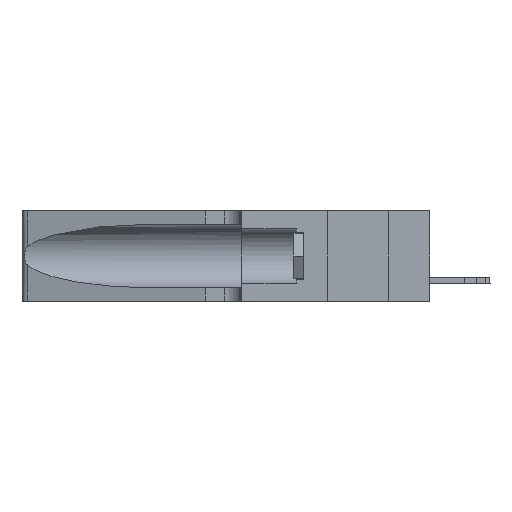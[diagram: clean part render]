
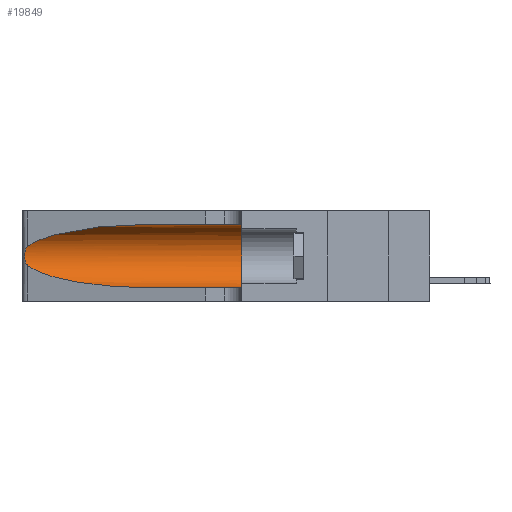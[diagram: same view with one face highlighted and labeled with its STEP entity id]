
A CAD part, left-side view. The second image highlights one B-rep face of the part: STEP entity #19849.
In plain terms, the highlighted cylindrical face has radius 3.308 mm (diameter 6.617 mm), a partial arc.
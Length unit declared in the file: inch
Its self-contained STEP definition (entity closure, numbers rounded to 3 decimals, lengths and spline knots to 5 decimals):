
#324 = CARTESIAN_POINT ( 'NONE',  ( 0.1305, 0.35, 0.31525 ) ) ;
#595 = CARTESIAN_POINT ( 'NONE',  ( 0.25856, 1.23593, 0.16098 ) ) ;
#1309 = CYLINDRICAL_SURFACE ( 'NONE', #14048, 0.13025 ) ;
#1411 = AXIS2_PLACEMENT_3D ( 'NONE', #2124, #25890, #4333 ) ;
#1624 = EDGE_CURVE ( 'NONE', #9108, #6388, #1844, .T. ) ;
#1844 = CIRCLE ( 'NONE', #1411, 0.13025 ) ;
#2124 = CARTESIAN_POINT ( 'NONE',  ( 0.1305, 0.35, 0.185 ) ) ;
#2140 = EDGE_CURVE ( 'NONE', #6096, #9663, #15116, .T. ) ;
#2176 = EDGE_CURVE ( 'NONE', #9663, #3178, #10924, .T. ) ;
#2189 = CARTESIAN_POINT ( 'NONE',  ( 0.1305, 0.72297, 0.05475 ) ) ;
#2686 = CARTESIAN_POINT ( 'NONE',  ( 0.25555, 1.22994, 0.2215 ) ) ;
#3178 = VERTEX_POINT ( 'NONE', #6890 ) ;
#3411 = CARTESIAN_POINT ( 'NONE',  ( 0.1305, 0.72297, 0.31525 ) ) ;
#4243 = EDGE_LOOP ( 'NONE', ( #12942, #7270, #9616, #6047, #6222, #5511 ) ) ;
#4333 = DIRECTION ( 'NONE',  ( 0., 0., 1. ) ) ;
#5511 = ORIENTED_EDGE ( 'NONE', *, *, #11638, .F. ) ;
#5536 = CARTESIAN_POINT ( 'NONE',  ( 0.25487, 1.22718, 0.14631 ) ) ;
#5581 = CARTESIAN_POINT ( 'NONE',  ( 0.25487, 1.22718, 0.22369 ) ) ;
#5882 = DIRECTION ( 'NONE',  ( 0., -1., 0. ) ) ;
#6047 = ORIENTED_EDGE ( 'NONE', *, *, #19781, .T. ) ;
#6096 = VERTEX_POINT ( 'NONE', #26958 ) ;
#6222 = ORIENTED_EDGE ( 'NONE', *, *, #1624, .F. ) ;
#6262 = LINE ( 'NONE', #22998, #12085 ) ;
#6388 = VERTEX_POINT ( 'NONE', #21529 ) ;
#6890 = CARTESIAN_POINT ( 'NONE',  ( 0.1305, 0.72297, 0.05475 ) ) ;
#6979 = CARTESIAN_POINT ( 'NONE',  ( 0.25787, 1.23484, 0.2124 ) ) ;
#7270 = ORIENTED_EDGE ( 'NONE', *, *, #2140, .T. ) ;
#8860 = VECTOR ( 'NONE', #16070, 39.37008 ) ;
#9083 = CARTESIAN_POINT ( 'NONE',  ( 0.26075, 1.23896, 0.178 ) ) ;
#9108 = VERTEX_POINT ( 'NONE', #324 ) ;
#9275 = CARTESIAN_POINT ( 'NONE',  ( 0.25555, 1.22993, 0.14849 ) ) ;
#9616 = ORIENTED_EDGE ( 'NONE', *, *, #2176, .T. ) ;
#9663 = VERTEX_POINT ( 'NONE', #13551 ) ;
#10099 = CARTESIAN_POINT ( 'NONE',  ( 0.18966, 0.96281, 0.05475 ) ) ;
#10146 = CARTESIAN_POINT ( 'NONE',  ( 0.2373, 1.15595, 0.28018 ) ) ;
#10924 =( BOUNDED_CURVE ( )  B_SPLINE_CURVE ( 3, ( #5536, #27480, #10099, #2189 ),
 .UNSPECIFIED., .F., .T. ) 
 B_SPLINE_CURVE_WITH_KNOTS ( ( 4, 4 ),
 ( 3.44316, 4.71239 ),
 .UNSPECIFIED. ) 
 CURVE ( )  GEOMETRIC_REPRESENTATION_ITEM ( )  RATIONAL_B_SPLINE_CURVE ( ( 1., 0.87, 0.87, 1. ) ) 
 REPRESENTATION_ITEM ( '' )  );
#11380 = CARTESIAN_POINT ( 'NONE',  ( 0.25487, 1.22718, 0.14631 ) ) ;
#11638 = EDGE_CURVE ( 'NONE', #19638, #9108, #6262, .T. ) ;
#12085 = VECTOR ( 'NONE', #5882, 39.37008 ) ;
#12942 = ORIENTED_EDGE ( 'NONE', *, *, #17885, .T. ) ;
#13419 = CARTESIAN_POINT ( 'NONE',  ( 0.1305, 1.61858, 0.185 ) ) ;
#13456 = CARTESIAN_POINT ( 'NONE',  ( 0.26075, 1.23896, 0.19203 ) ) ;
#13551 = CARTESIAN_POINT ( 'NONE',  ( 0.25487, 1.22718, 0.14631 ) ) ;
#13652 = CARTESIAN_POINT ( 'NONE',  ( 0.26017, 1.23833, 0.17102 ) ) ;
#13742 = CARTESIAN_POINT ( 'NONE',  ( 0.25639, 1.23184, 0.21858 ) ) ;
#14048 = AXIS2_PLACEMENT_3D ( 'NONE', #13419, #26315, #24207 ) ;
#15116 = B_SPLINE_CURVE_WITH_KNOTS ( 'NONE', 3,
 ( #20219, #2686, #13742, #6979, #15669, #15569, #13456, #9083, #13652, #595, #24329, #17852, #9275, #11380 ),
 .UNSPECIFIED., .F., .F.,
 ( 4, 2, 2, 2, 2, 2, 4 ),
 ( 0., 0.00027, 0.00053, 0.00107, 0.0016, 0.00187, 0.00214 ),
 .UNSPECIFIED. ) ;
#15569 = CARTESIAN_POINT ( 'NONE',  ( 0.26018, 1.23835, 0.19895 ) ) ;
#15669 = CARTESIAN_POINT ( 'NONE',  ( 0.25854, 1.2359, 0.20912 ) ) ;
#16070 = DIRECTION ( 'NONE',  ( 0., -1., 0. ) ) ;
#16358 = LINE ( 'NONE', #26387, #8860 ) ;
#16734 = CARTESIAN_POINT ( 'NONE',  ( 0.1305, 0.72297, 0.31525 ) ) ;
#17852 = CARTESIAN_POINT ( 'NONE',  ( 0.25639, 1.23186, 0.15144 ) ) ;
#17885 = EDGE_CURVE ( 'NONE', #19638, #6096, #24892, .T. ) ;
#19638 = VERTEX_POINT ( 'NONE', #3411 ) ;
#19781 = EDGE_CURVE ( 'NONE', #3178, #6388, #16358, .T. ) ;
#19849 = ADVANCED_FACE ( 'NONE', ( #21465 ), #1309, .F. ) ;
#20219 = CARTESIAN_POINT ( 'NONE',  ( 0.25487, 1.22718, 0.22369 ) ) ;
#21465 = FACE_OUTER_BOUND ( 'NONE', #4243, .T. ) ;
#21529 = CARTESIAN_POINT ( 'NONE',  ( 0.1305, 0.35, 0.05475 ) ) ;
#22998 = CARTESIAN_POINT ( 'NONE',  ( 0.1305, 1.61858, 0.31525 ) ) ;
#24207 = DIRECTION ( 'NONE',  ( 0., 0., -1. ) ) ;
#24329 = CARTESIAN_POINT ( 'NONE',  ( 0.25789, 1.23486, 0.15765 ) ) ;
#24892 =( BOUNDED_CURVE ( )  B_SPLINE_CURVE ( 3, ( #16734, #27417, #10146, #5581 ),
 .UNSPECIFIED., .F., .T. ) 
 B_SPLINE_CURVE_WITH_KNOTS ( ( 4, 4 ),
 ( 1.5708, 2.84003 ),
 .UNSPECIFIED. ) 
 CURVE ( )  GEOMETRIC_REPRESENTATION_ITEM ( )  RATIONAL_B_SPLINE_CURVE ( ( 1., 0.87, 0.87, 1. ) ) 
 REPRESENTATION_ITEM ( '' )  );
#25890 = DIRECTION ( 'NONE',  ( 0., 1., 0. ) ) ;
#26315 = DIRECTION ( 'NONE',  ( 0., -1., 0. ) ) ;
#26387 = CARTESIAN_POINT ( 'NONE',  ( 0.1305, 1.61858, 0.05475 ) ) ;
#26958 = CARTESIAN_POINT ( 'NONE',  ( 0.25487, 1.22718, 0.22369 ) ) ;
#27417 = CARTESIAN_POINT ( 'NONE',  ( 0.18966, 0.96281, 0.31525 ) ) ;
#27480 = CARTESIAN_POINT ( 'NONE',  ( 0.2373, 1.15595, 0.08982 ) ) ;
